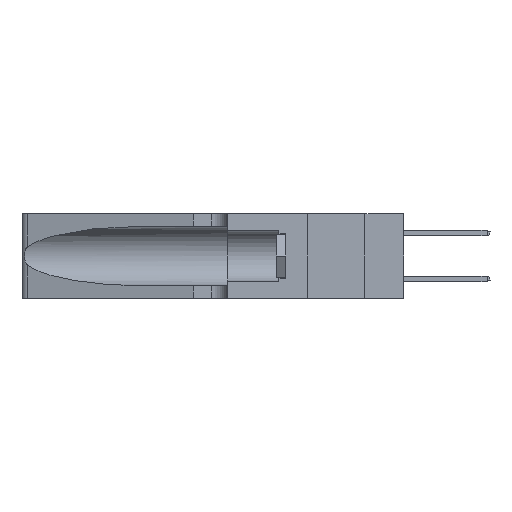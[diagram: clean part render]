
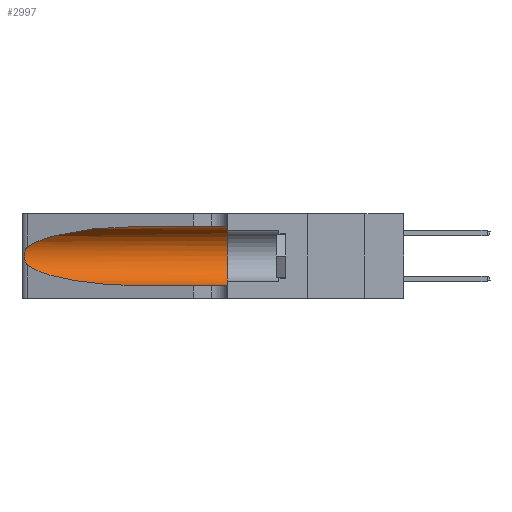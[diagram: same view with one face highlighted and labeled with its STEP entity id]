
A CAD part, left-side view. The second image highlights one B-rep face of the part: STEP entity #2997.
In plain terms, the highlighted cylindrical face has radius 3.308 mm (diameter 6.617 mm), a partial arc.
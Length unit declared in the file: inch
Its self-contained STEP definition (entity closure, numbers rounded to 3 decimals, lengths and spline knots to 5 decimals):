
#24 = DIRECTION ( 'NONE',  ( 0., 0., 1. ) ) ;
#824 = VERTEX_POINT ( 'NONE', #8848 ) ;
#1165 = ORIENTED_EDGE ( 'NONE', *, *, #13935, .T. ) ;
#1665 = CARTESIAN_POINT ( 'NONE',  ( 0.25856, 1.23593, 0.16098 ) ) ;
#1723 = DIRECTION ( 'NONE',  ( 0., -1., 0. ) ) ;
#1792 = CARTESIAN_POINT ( 'NONE',  ( 0.1305, 0.72297, 0.31525 ) ) ;
#1847 = VERTEX_POINT ( 'NONE', #17877 ) ;
#1865 = CARTESIAN_POINT ( 'NONE',  ( 0.25487, 1.22718, 0.22369 ) ) ;
#2215 = CIRCLE ( 'NONE', #14782, 0.13025 ) ;
#2920 = CYLINDRICAL_SURFACE ( 'NONE', #6513, 0.13025 ) ;
#2997 = ADVANCED_FACE ( 'NONE', ( #11864 ), #2920, .F. ) ;
#3025 = B_SPLINE_CURVE_WITH_KNOTS ( 'NONE', 3,
 ( #5015, #13379, #6731, #18362, #8427, #20004, #10116, #21631, #11769, #1665, #13454, #3409, #15118, #5099 ),
 .UNSPECIFIED., .F., .F.,
 ( 4, 2, 2, 2, 2, 2, 4 ),
 ( 0., 0.00027, 0.00053, 0.00107, 0.0016, 0.00187, 0.00214 ),
 .UNSPECIFIED. ) ;
#3178 =( BOUNDED_CURVE ( )  B_SPLINE_CURVE ( 3, ( #1792, #15243, #11975, #1865 ),
 .UNSPECIFIED., .F., .F. ) 
 B_SPLINE_CURVE_WITH_KNOTS ( ( 4, 4 ),
 ( 1.5708, 2.84003 ),
 .UNSPECIFIED. ) 
 CURVE ( )  GEOMETRIC_REPRESENTATION_ITEM ( )  RATIONAL_B_SPLINE_CURVE ( ( 1., 0.87, 0.87, 1. ) ) 
 REPRESENTATION_ITEM ( '' )  );
#3235 = CARTESIAN_POINT ( 'NONE',  ( 0.18966, 0.96281, 0.05475 ) ) ;
#3409 = CARTESIAN_POINT ( 'NONE',  ( 0.25639, 1.23186, 0.15144 ) ) ;
#3648 = LINE ( 'NONE', #11826, #12557 ) ;
#4247 =( BOUNDED_CURVE ( )  B_SPLINE_CURVE ( 3, ( #21465, #19835, #3235, #14942 ),
 .UNSPECIFIED., .F., .T. ) 
 B_SPLINE_CURVE_WITH_KNOTS ( ( 4, 4 ),
 ( 3.44316, 4.71239 ),
 .UNSPECIFIED. ) 
 CURVE ( )  GEOMETRIC_REPRESENTATION_ITEM ( )  RATIONAL_B_SPLINE_CURVE ( ( 1., 0.87, 0.87, 1. ) ) 
 REPRESENTATION_ITEM ( '' )  );
#4282 = VECTOR ( 'NONE', #18446, 39.37008 ) ;
#5015 = CARTESIAN_POINT ( 'NONE',  ( 0.25487, 1.22718, 0.22369 ) ) ;
#5099 = CARTESIAN_POINT ( 'NONE',  ( 0.25487, 1.22718, 0.14631 ) ) ;
#5791 = EDGE_CURVE ( 'NONE', #17474, #1847, #3648, .T. ) ;
#5822 = VERTEX_POINT ( 'NONE', #8792 ) ;
#6186 = CARTESIAN_POINT ( 'NONE',  ( 0.1305, 0.72297, 0.31525 ) ) ;
#6513 = AXIS2_PLACEMENT_3D ( 'NONE', #19435, #12792, #7842 ) ;
#6669 = CARTESIAN_POINT ( 'NONE',  ( 0.25487, 1.22718, 0.22369 ) ) ;
#6731 = CARTESIAN_POINT ( 'NONE',  ( 0.25639, 1.23184, 0.21858 ) ) ;
#7842 = DIRECTION ( 'NONE',  ( 0., 0., -1. ) ) ;
#8084 = EDGE_LOOP ( 'NONE', ( #1165, #16565, #13874, #11849, #19135, #19944 ) ) ;
#8375 = EDGE_CURVE ( 'NONE', #18038, #824, #4247, .T. ) ;
#8427 = CARTESIAN_POINT ( 'NONE',  ( 0.25854, 1.2359, 0.20912 ) ) ;
#8433 = CARTESIAN_POINT ( 'NONE',  ( 0.1305, 1.61858, 0.05475 ) ) ;
#8781 = LINE ( 'NONE', #8433, #4282 ) ;
#8792 = CARTESIAN_POINT ( 'NONE',  ( 0.1305, 0.35, 0.05475 ) ) ;
#8848 = CARTESIAN_POINT ( 'NONE',  ( 0.1305, 0.72297, 0.05475 ) ) ;
#10116 = CARTESIAN_POINT ( 'NONE',  ( 0.26075, 1.23896, 0.19203 ) ) ;
#10191 = DIRECTION ( 'NONE',  ( 0., 1., 0. ) ) ;
#11268 = EDGE_CURVE ( 'NONE', #1847, #5822, #2215, .T. ) ;
#11769 = CARTESIAN_POINT ( 'NONE',  ( 0.26017, 1.23833, 0.17102 ) ) ;
#11826 = CARTESIAN_POINT ( 'NONE',  ( 0.1305, 1.61858, 0.31525 ) ) ;
#11849 = ORIENTED_EDGE ( 'NONE', *, *, #13163, .T. ) ;
#11864 = FACE_OUTER_BOUND ( 'NONE', #8084, .T. ) ;
#11975 = CARTESIAN_POINT ( 'NONE',  ( 0.2373, 1.15595, 0.28018 ) ) ;
#12557 = VECTOR ( 'NONE', #1723, 39.37008 ) ;
#12792 = DIRECTION ( 'NONE',  ( 0., -1., 0. ) ) ;
#13102 = VERTEX_POINT ( 'NONE', #6669 ) ;
#13163 = EDGE_CURVE ( 'NONE', #824, #5822, #8781, .T. ) ;
#13379 = CARTESIAN_POINT ( 'NONE',  ( 0.25555, 1.22994, 0.2215 ) ) ;
#13454 = CARTESIAN_POINT ( 'NONE',  ( 0.25789, 1.23486, 0.15765 ) ) ;
#13874 = ORIENTED_EDGE ( 'NONE', *, *, #8375, .T. ) ;
#13935 = EDGE_CURVE ( 'NONE', #17474, #13102, #3178, .T. ) ;
#14782 = AXIS2_PLACEMENT_3D ( 'NONE', #20083, #10191, #24 ) ;
#14942 = CARTESIAN_POINT ( 'NONE',  ( 0.1305, 0.72297, 0.05475 ) ) ;
#15118 = CARTESIAN_POINT ( 'NONE',  ( 0.25555, 1.22993, 0.14849 ) ) ;
#15243 = CARTESIAN_POINT ( 'NONE',  ( 0.18966, 0.96281, 0.31525 ) ) ;
#15931 = EDGE_CURVE ( 'NONE', #13102, #18038, #3025, .T. ) ;
#16565 = ORIENTED_EDGE ( 'NONE', *, *, #15931, .T. ) ;
#17474 = VERTEX_POINT ( 'NONE', #6186 ) ;
#17877 = CARTESIAN_POINT ( 'NONE',  ( 0.1305, 0.35, 0.31525 ) ) ;
#18038 = VERTEX_POINT ( 'NONE', #19242 ) ;
#18362 = CARTESIAN_POINT ( 'NONE',  ( 0.25787, 1.23484, 0.2124 ) ) ;
#18446 = DIRECTION ( 'NONE',  ( 0., -1., 0. ) ) ;
#19135 = ORIENTED_EDGE ( 'NONE', *, *, #11268, .F. ) ;
#19242 = CARTESIAN_POINT ( 'NONE',  ( 0.25487, 1.22718, 0.14631 ) ) ;
#19435 = CARTESIAN_POINT ( 'NONE',  ( 0.1305, 1.61858, 0.185 ) ) ;
#19835 = CARTESIAN_POINT ( 'NONE',  ( 0.2373, 1.15595, 0.08982 ) ) ;
#19944 = ORIENTED_EDGE ( 'NONE', *, *, #5791, .F. ) ;
#20004 = CARTESIAN_POINT ( 'NONE',  ( 0.26018, 1.23835, 0.19895 ) ) ;
#20083 = CARTESIAN_POINT ( 'NONE',  ( 0.1305, 0.35, 0.185 ) ) ;
#21465 = CARTESIAN_POINT ( 'NONE',  ( 0.25487, 1.22718, 0.14631 ) ) ;
#21631 = CARTESIAN_POINT ( 'NONE',  ( 0.26075, 1.23896, 0.178 ) ) ;
